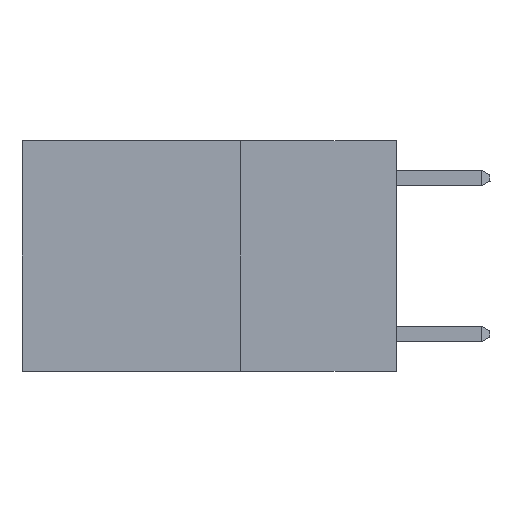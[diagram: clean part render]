
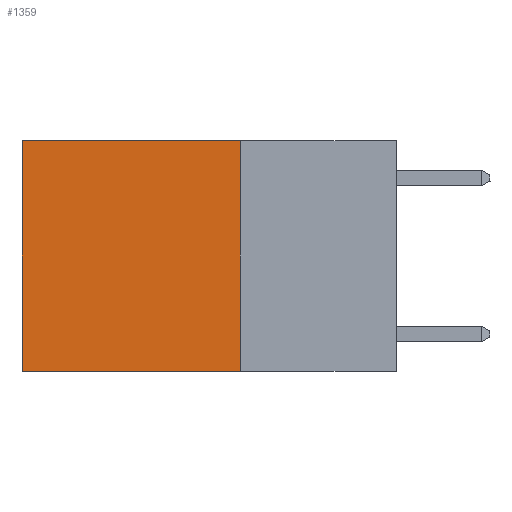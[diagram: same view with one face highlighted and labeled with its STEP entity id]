
A CAD part, left-side view. The second image highlights one B-rep face of the part: STEP entity #1359.
In plain terms, the highlighted planar face has unit normal (-1, 0, 0).
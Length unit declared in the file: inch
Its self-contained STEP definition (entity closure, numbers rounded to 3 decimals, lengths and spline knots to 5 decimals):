
#1078 = FACE_OUTER_BOUND ( 'NONE', #2109, .T. ) ;
#1359 = ADVANCED_FACE ( 'NONE', ( #1078 ), #9825, .F. ) ;
#2109 = EDGE_LOOP ( 'NONE', ( #10011, #3750, #11060, #8003 ) ) ;
#2597 = DIRECTION ( 'NONE',  ( 1., 0., 0. ) ) ;
#3336 = EDGE_CURVE ( 'NONE', #10603, #15617, #8589, .T. ) ;
#3750 = ORIENTED_EDGE ( 'NONE', *, *, #3336, .F. ) ;
#3963 = EDGE_CURVE ( 'NONE', #4581, #10603, #18225, .T. ) ;
#4581 = VERTEX_POINT ( 'NONE', #21468 ) ;
#8003 = ORIENTED_EDGE ( 'NONE', *, *, #10840, .T. ) ;
#8530 = DIRECTION ( 'NONE',  ( 0., 1., 0. ) ) ;
#8589 = LINE ( 'NONE', #23231, #16075 ) ;
#8825 = EDGE_CURVE ( 'NONE', #19446, #15617, #23668, .T. ) ;
#9279 = VECTOR ( 'NONE', #25183, 39.37008 ) ;
#9697 = DIRECTION ( 'NONE',  ( 0., 0., -1. ) ) ;
#9825 = PLANE ( 'NONE',  #20935 ) ;
#10011 = ORIENTED_EDGE ( 'NONE', *, *, #8825, .T. ) ;
#10603 = VERTEX_POINT ( 'NONE', #12297 ) ;
#10840 = EDGE_CURVE ( 'NONE', #4581, #19446, #11223, .T. ) ;
#11060 = ORIENTED_EDGE ( 'NONE', *, *, #3963, .F. ) ;
#11223 = LINE ( 'NONE', #16380, #21556 ) ;
#12297 = CARTESIAN_POINT ( 'NONE',  ( 0.2625, 0.25, -0.37 ) ) ;
#12914 = VECTOR ( 'NONE', #9697, 39.37008 ) ;
#13051 = CARTESIAN_POINT ( 'NONE',  ( 0.2625, 0.6, -0.37 ) ) ;
#15617 = VERTEX_POINT ( 'NONE', #13051 ) ;
#15894 = CARTESIAN_POINT ( 'NONE',  ( 0.2625, 0.25, 0. ) ) ;
#16075 = VECTOR ( 'NONE', #18925, 39.37008 ) ;
#16380 = CARTESIAN_POINT ( 'NONE',  ( 0.2625, 0.25, 0. ) ) ;
#17940 = CARTESIAN_POINT ( 'NONE',  ( 0.2625, 0.25, 0. ) ) ;
#18225 = LINE ( 'NONE', #15894, #12914 ) ;
#18925 = DIRECTION ( 'NONE',  ( 0., 1., 0. ) ) ;
#19446 = VERTEX_POINT ( 'NONE', #25588 ) ;
#20935 = AXIS2_PLACEMENT_3D ( 'NONE', #17940, #2597, #24536 ) ;
#20949 = CARTESIAN_POINT ( 'NONE',  ( 0.2625, 0.6, 0. ) ) ;
#21468 = CARTESIAN_POINT ( 'NONE',  ( 0.2625, 0.25, 0. ) ) ;
#21556 = VECTOR ( 'NONE', #8530, 39.37008 ) ;
#23231 = CARTESIAN_POINT ( 'NONE',  ( 0.2625, 0.25, -0.37 ) ) ;
#23668 = LINE ( 'NONE', #20949, #9279 ) ;
#24536 = DIRECTION ( 'NONE',  ( 0., 0., -1. ) ) ;
#25183 = DIRECTION ( 'NONE',  ( 0., 0., -1. ) ) ;
#25588 = CARTESIAN_POINT ( 'NONE',  ( 0.2625, 0.6, 0. ) ) ;
